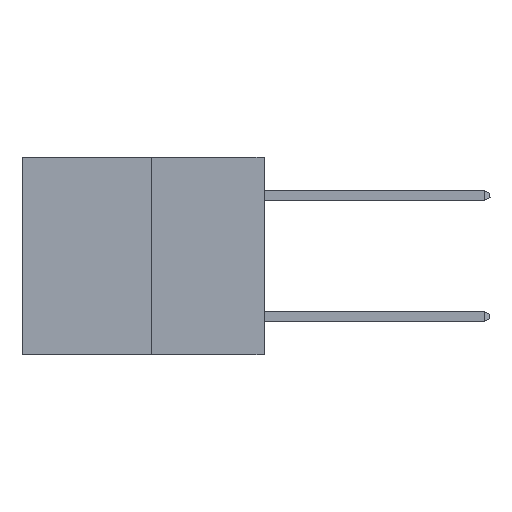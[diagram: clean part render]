
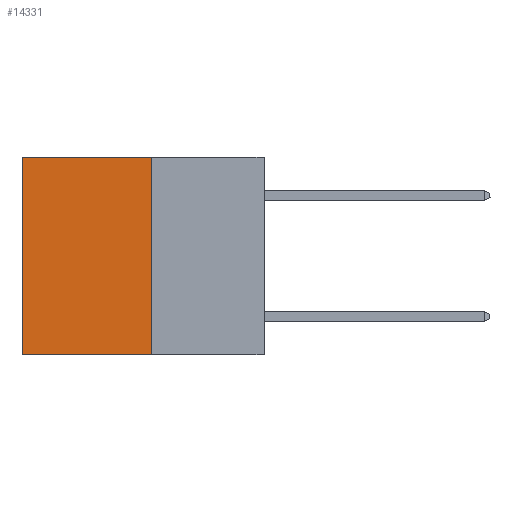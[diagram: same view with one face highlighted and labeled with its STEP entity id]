
A CAD part, left-side view. The second image highlights one B-rep face of the part: STEP entity #14331.
In plain terms, the highlighted planar face has unit normal (-1, 0, 0).
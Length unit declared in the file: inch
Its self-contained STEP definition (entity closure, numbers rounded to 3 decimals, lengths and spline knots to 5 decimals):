
#433 = VECTOR ( 'NONE', #13923, 39.37008 ) ;
#729 = ORIENTED_EDGE ( 'NONE', *, *, #19217, .F. ) ;
#2207 = DIRECTION ( 'NONE',  ( 0., 0., -1. ) ) ;
#2407 = CARTESIAN_POINT ( 'NONE',  ( 0.3165, 0.28, 0. ) ) ;
#2436 = CARTESIAN_POINT ( 'NONE',  ( 0.3165, 0.6, -0.49 ) ) ;
#2475 = CARTESIAN_POINT ( 'NONE',  ( 0.3165, 0.6, 0. ) ) ;
#2614 = VERTEX_POINT ( 'NONE', #20825 ) ;
#3038 = CARTESIAN_POINT ( 'NONE',  ( 0.3165, 0.28, 0. ) ) ;
#3807 = EDGE_CURVE ( 'NONE', #21298, #2614, #21303, .T. ) ;
#4065 = ORIENTED_EDGE ( 'NONE', *, *, #15288, .T. ) ;
#4256 = AXIS2_PLACEMENT_3D ( 'NONE', #9308, #21519, #11146 ) ;
#4300 = VERTEX_POINT ( 'NONE', #2475 ) ;
#5242 = CARTESIAN_POINT ( 'NONE',  ( 0.3165, 0.28, -0.49 ) ) ;
#8273 = EDGE_LOOP ( 'NONE', ( #16552, #729, #19537, #4065 ) ) ;
#8693 = CARTESIAN_POINT ( 'NONE',  ( 0.3165, 0.28, -0.49 ) ) ;
#9308 = CARTESIAN_POINT ( 'NONE',  ( 0.3165, 0.28, -0.49 ) ) ;
#11146 = DIRECTION ( 'NONE',  ( 0., 0., -1. ) ) ;
#11307 = VECTOR ( 'NONE', #14467, 39.37008 ) ;
#13025 = VECTOR ( 'NONE', #18986, 39.37008 ) ;
#13923 = DIRECTION ( 'NONE',  ( 0., 0., -1. ) ) ;
#14331 = ADVANCED_FACE ( 'NONE', ( #20871 ), #18164, .F. ) ;
#14467 = DIRECTION ( 'NONE',  ( 0., 1., 0. ) ) ;
#14782 = EDGE_CURVE ( 'NONE', #4300, #15641, #16736, .T. ) ;
#15288 = EDGE_CURVE ( 'NONE', #21298, #4300, #21865, .T. ) ;
#15641 = VERTEX_POINT ( 'NONE', #20286 ) ;
#15672 = VECTOR ( 'NONE', #2207, 39.37008 ) ;
#16552 = ORIENTED_EDGE ( 'NONE', *, *, #14782, .T. ) ;
#16736 = LINE ( 'NONE', #2436, #15672 ) ;
#17074 = LINE ( 'NONE', #5242, #13025 ) ;
#18164 = PLANE ( 'NONE',  #4256 ) ;
#18986 = DIRECTION ( 'NONE',  ( 0., 1., 0. ) ) ;
#19217 = EDGE_CURVE ( 'NONE', #2614, #15641, #17074, .T. ) ;
#19537 = ORIENTED_EDGE ( 'NONE', *, *, #3807, .F. ) ;
#20286 = CARTESIAN_POINT ( 'NONE',  ( 0.3165, 0.6, -0.49 ) ) ;
#20825 = CARTESIAN_POINT ( 'NONE',  ( 0.3165, 0.28, -0.49 ) ) ;
#20871 = FACE_OUTER_BOUND ( 'NONE', #8273, .T. ) ;
#21298 = VERTEX_POINT ( 'NONE', #3038 ) ;
#21303 = LINE ( 'NONE', #8693, #433 ) ;
#21519 = DIRECTION ( 'NONE',  ( 1., 0., 0. ) ) ;
#21865 = LINE ( 'NONE', #2407, #11307 ) ;
